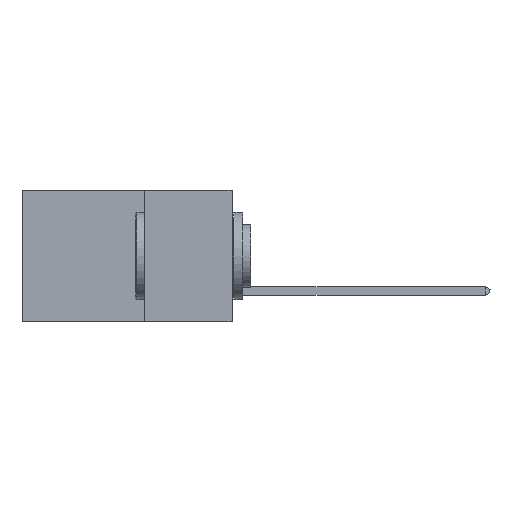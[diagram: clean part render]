
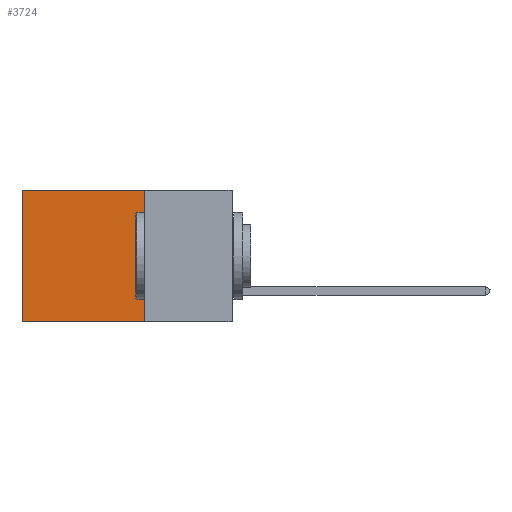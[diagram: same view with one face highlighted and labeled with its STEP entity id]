
A CAD part, left-side view. The second image highlights one B-rep face of the part: STEP entity #3724.
In plain terms, the highlighted planar face has unit normal (-1, 0, 0).
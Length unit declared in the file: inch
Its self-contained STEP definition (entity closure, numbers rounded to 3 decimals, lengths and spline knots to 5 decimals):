
#201 = VECTOR ( 'NONE', #12132, 39.37008 ) ;
#329 = EDGE_CURVE ( 'NONE', #12186, #1901, #5713, .T. ) ;
#681 = EDGE_CURVE ( 'NONE', #2201, #6134, #5953, .T. ) ;
#840 = CARTESIAN_POINT ( 'NONE',  ( 0.2875, 0.6, -0.375 ) ) ;
#1730 = DIRECTION ( 'NONE',  ( 0., 1., 0. ) ) ;
#1886 = DIRECTION ( 'NONE',  ( 1., 0., 0. ) ) ;
#1901 = VERTEX_POINT ( 'NONE', #3028 ) ;
#2108 = DIRECTION ( 'NONE',  ( 0., 1., 0. ) ) ;
#2201 = VERTEX_POINT ( 'NONE', #5795 ) ;
#2205 = AXIS2_PLACEMENT_3D ( 'NONE', #7194, #1886, #10633 ) ;
#3028 = CARTESIAN_POINT ( 'NONE',  ( 0.2875, 0.25, -0.375 ) ) ;
#3460 = ORIENTED_EDGE ( 'NONE', *, *, #681, .T. ) ;
#3724 = ADVANCED_FACE ( 'NONE', ( #5331 ), #12722, .F. ) ;
#3848 = EDGE_CURVE ( 'NONE', #12186, #2201, #9447, .T. ) ;
#4054 = VECTOR ( 'NONE', #2108, 39.37008 ) ;
#5308 = ORIENTED_EDGE ( 'NONE', *, *, #329, .F. ) ;
#5331 = FACE_OUTER_BOUND ( 'NONE', #13293, .T. ) ;
#5484 = ORIENTED_EDGE ( 'NONE', *, *, #8154, .F. ) ;
#5713 = LINE ( 'NONE', #8924, #201 ) ;
#5795 = CARTESIAN_POINT ( 'NONE',  ( 0.2875, 0.6, 0. ) ) ;
#5905 = VECTOR ( 'NONE', #1730, 39.37008 ) ;
#5953 = LINE ( 'NONE', #840, #12739 ) ;
#5996 = CARTESIAN_POINT ( 'NONE',  ( 0.2875, 0.25, -0.375 ) ) ;
#6134 = VERTEX_POINT ( 'NONE', #10221 ) ;
#6996 = DIRECTION ( 'NONE',  ( 0., 0., -1. ) ) ;
#7194 = CARTESIAN_POINT ( 'NONE',  ( 0.2875, 0.25, -0.375 ) ) ;
#7703 = ORIENTED_EDGE ( 'NONE', *, *, #3848, .T. ) ;
#8154 = EDGE_CURVE ( 'NONE', #1901, #6134, #12429, .T. ) ;
#8924 = CARTESIAN_POINT ( 'NONE',  ( 0.2875, 0.25, -0.375 ) ) ;
#9447 = LINE ( 'NONE', #13705, #4054 ) ;
#10221 = CARTESIAN_POINT ( 'NONE',  ( 0.2875, 0.6, -0.375 ) ) ;
#10633 = DIRECTION ( 'NONE',  ( 0., 0., -1. ) ) ;
#10798 = CARTESIAN_POINT ( 'NONE',  ( 0.2875, 0.25, 0. ) ) ;
#12132 = DIRECTION ( 'NONE',  ( 0., 0., -1. ) ) ;
#12186 = VERTEX_POINT ( 'NONE', #10798 ) ;
#12429 = LINE ( 'NONE', #5996, #5905 ) ;
#12722 = PLANE ( 'NONE',  #2205 ) ;
#12739 = VECTOR ( 'NONE', #6996, 39.37008 ) ;
#13293 = EDGE_LOOP ( 'NONE', ( #3460, #5484, #5308, #7703 ) ) ;
#13705 = CARTESIAN_POINT ( 'NONE',  ( 0.2875, 0.25, 0. ) ) ;
